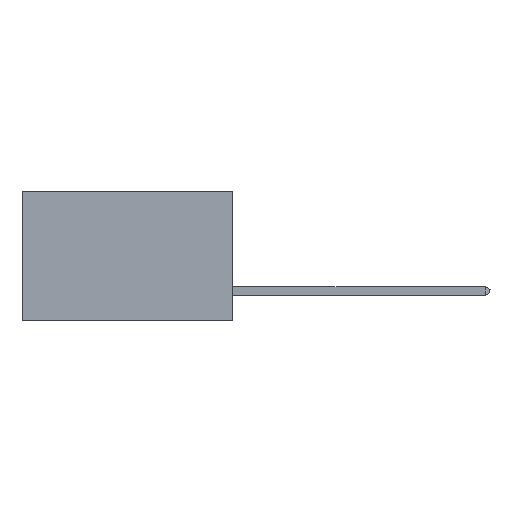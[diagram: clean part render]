
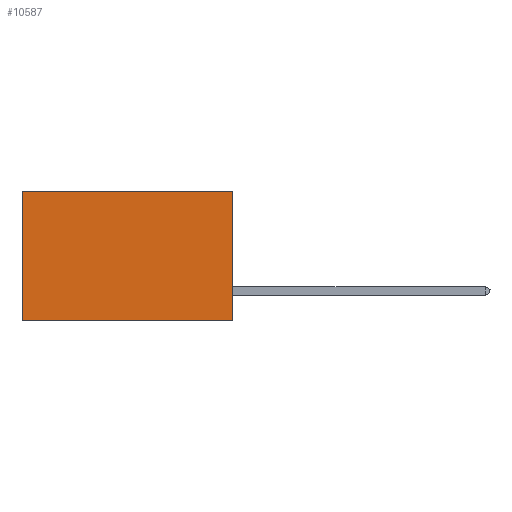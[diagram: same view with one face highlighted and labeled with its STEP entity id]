
A CAD part, left-side view. The second image highlights one B-rep face of the part: STEP entity #10587.
In plain terms, the highlighted planar face has unit normal (-1, 0, 0).
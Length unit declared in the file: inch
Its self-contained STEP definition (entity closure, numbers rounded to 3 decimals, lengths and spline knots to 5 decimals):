
#934 = CARTESIAN_POINT ( 'NONE',  ( 0.2875, 0.6, -0.37 ) ) ;
#1433 = CARTESIAN_POINT ( 'NONE',  ( 0.2875, 0., 0. ) ) ;
#2220 = LINE ( 'NONE', #19364, #18421 ) ;
#2474 = EDGE_CURVE ( 'NONE', #33089, #11146, #16656, .T. ) ;
#8281 = CARTESIAN_POINT ( 'NONE',  ( 0.2875, 0.6, 0. ) ) ;
#9099 = DIRECTION ( 'NONE',  ( 0., 1., 0. ) ) ;
#10587 = ADVANCED_FACE ( 'NONE', ( #41935 ), #43561, .F. ) ;
#10628 = LINE ( 'NONE', #19876, #29062 ) ;
#11146 = VERTEX_POINT ( 'NONE', #934 ) ;
#12188 = VERTEX_POINT ( 'NONE', #32868 ) ;
#12322 = VECTOR ( 'NONE', #38404, 39.37008 ) ;
#12395 = ORIENTED_EDGE ( 'NONE', *, *, #46755, .T. ) ;
#14492 = DIRECTION ( 'NONE',  ( 0., 1., 0. ) ) ;
#16545 = AXIS2_PLACEMENT_3D ( 'NONE', #43892, #25266, #25578 ) ;
#16656 = LINE ( 'NONE', #29181, #20086 ) ;
#18421 = VECTOR ( 'NONE', #44858, 39.37008 ) ;
#19364 = CARTESIAN_POINT ( 'NONE',  ( 0.2875, 0., 0. ) ) ;
#19876 = CARTESIAN_POINT ( 'NONE',  ( 0.2875, 0., 0. ) ) ;
#20086 = VECTOR ( 'NONE', #14492, 39.37008 ) ;
#21405 = CARTESIAN_POINT ( 'NONE',  ( 0.2875, 0., -0.37 ) ) ;
#22830 = EDGE_CURVE ( 'NONE', #39977, #33089, #2220, .T. ) ;
#25266 = DIRECTION ( 'NONE',  ( 1., 0., 0. ) ) ;
#25578 = DIRECTION ( 'NONE',  ( 0., 0., -1. ) ) ;
#29062 = VECTOR ( 'NONE', #9099, 39.37008 ) ;
#29181 = CARTESIAN_POINT ( 'NONE',  ( 0.2875, 0., -0.37 ) ) ;
#31945 = ORIENTED_EDGE ( 'NONE', *, *, #22830, .F. ) ;
#32868 = CARTESIAN_POINT ( 'NONE',  ( 0.2875, 0.6, 0. ) ) ;
#33089 = VERTEX_POINT ( 'NONE', #21405 ) ;
#33210 = LINE ( 'NONE', #8281, #12322 ) ;
#34032 = EDGE_LOOP ( 'NONE', ( #44073, #34124, #31945, #12395 ) ) ;
#34124 = ORIENTED_EDGE ( 'NONE', *, *, #2474, .F. ) ;
#38404 = DIRECTION ( 'NONE',  ( 0., 0., -1. ) ) ;
#39977 = VERTEX_POINT ( 'NONE', #1433 ) ;
#41935 = FACE_OUTER_BOUND ( 'NONE', #34032, .T. ) ;
#43561 = PLANE ( 'NONE',  #16545 ) ;
#43892 = CARTESIAN_POINT ( 'NONE',  ( 0.2875, 0., 0. ) ) ;
#44073 = ORIENTED_EDGE ( 'NONE', *, *, #45345, .T. ) ;
#44858 = DIRECTION ( 'NONE',  ( 0., 0., -1. ) ) ;
#45345 = EDGE_CURVE ( 'NONE', #12188, #11146, #33210, .T. ) ;
#46755 = EDGE_CURVE ( 'NONE', #39977, #12188, #10628, .T. ) ;
